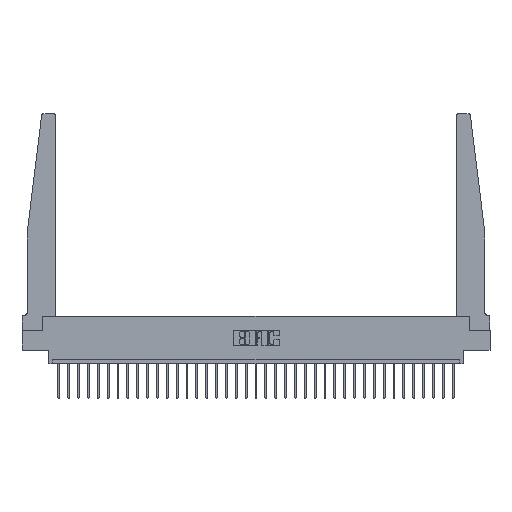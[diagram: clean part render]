
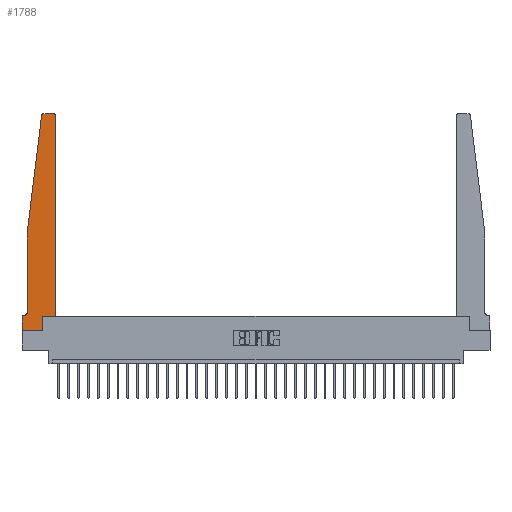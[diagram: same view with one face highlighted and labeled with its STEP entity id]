
A CAD part, top view. The second image highlights one B-rep face of the part: STEP entity #1788.
In plain terms, the highlighted planar face has unit normal (0, 0, 1).
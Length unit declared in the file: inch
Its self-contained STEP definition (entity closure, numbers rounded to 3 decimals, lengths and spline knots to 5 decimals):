
#302 = CARTESIAN_POINT ( 'NONE',  ( 0.065, 0.2375, 0.37 ) ) ;
#506 = DIRECTION ( 'NONE',  ( -0.122, -0.992, 0. ) ) ;
#744 = CARTESIAN_POINT ( 'NONE',  ( 0., 0.1875, 0.37 ) ) ;
#824 = ORIENTED_EDGE ( 'NONE', *, *, #11324, .T. ) ;
#980 = EDGE_LOOP ( 'NONE', ( #824, #16564, #9318, #1576, #23604, #6569, #13724, #20115, #16666, #25024, #13963, #1982 ) ) ;
#1576 = ORIENTED_EDGE ( 'NONE', *, *, #7150, .T. ) ;
#1788 = ADVANCED_FACE ( 'NONE', ( #30078 ), #11517, .T. ) ;
#1829 = EDGE_CURVE ( 'NONE', #10884, #9314, #3560, .T. ) ;
#1982 = ORIENTED_EDGE ( 'NONE', *, *, #28916, .T. ) ;
#1993 = CARTESIAN_POINT ( 'NONE',  ( 0.2605, 0.18, 0.37 ) ) ;
#2552 = VERTEX_POINT ( 'NONE', #6690 ) ;
#2892 = DIRECTION ( 'NONE',  ( -1., 0., 0. ) ) ;
#2907 = VECTOR ( 'NONE', #6822, 39.37008 ) ;
#3037 = VECTOR ( 'NONE', #506, 39.37008 ) ;
#3065 = CARTESIAN_POINT ( 'NONE',  ( 0.395, 2.72, 0.37 ) ) ;
#3560 = LINE ( 'NONE', #10199, #16468 ) ;
#4560 = CARTESIAN_POINT ( 'NONE',  ( 0.24675, 2.72367, 0.37 ) ) ;
#4687 = AXIS2_PLACEMENT_3D ( 'NONE', #11309, #6859, #18734 ) ;
#6132 = VERTEX_POINT ( 'NONE', #302 ) ;
#6374 = CARTESIAN_POINT ( 'NONE',  ( 0.27653, 2.75, 0.37 ) ) ;
#6459 = DIRECTION ( 'NONE',  ( 0., 0., 1. ) ) ;
#6569 = ORIENTED_EDGE ( 'NONE', *, *, #26447, .T. ) ;
#6690 = CARTESIAN_POINT ( 'NONE',  ( 0.395, 2.75, 0.37 ) ) ;
#6822 = DIRECTION ( 'NONE',  ( 1., 0., 0. ) ) ;
#6859 = DIRECTION ( 'NONE',  ( 0., 0., 1. ) ) ;
#6963 = VECTOR ( 'NONE', #16775, 39.37008 ) ;
#7150 = EDGE_CURVE ( 'NONE', #11729, #6132, #19220, .T. ) ;
#7693 = DIRECTION ( 'NONE',  ( 0., 0., -1. ) ) ;
#7741 = CIRCLE ( 'NONE', #8995, 0.03 ) ;
#8168 = LINE ( 'NONE', #14365, #14815 ) ;
#8438 = VERTEX_POINT ( 'NONE', #744 ) ;
#8867 = VECTOR ( 'NONE', #28733, 39.37008 ) ;
#8995 = AXIS2_PLACEMENT_3D ( 'NONE', #3065, #21773, #28898 ) ;
#9023 = CARTESIAN_POINT ( 'NONE',  ( 0.015, 0.1875, 0.37 ) ) ;
#9314 = VERTEX_POINT ( 'NONE', #27834 ) ;
#9318 = ORIENTED_EDGE ( 'NONE', *, *, #17857, .T. ) ;
#10199 = CARTESIAN_POINT ( 'NONE',  ( 0., 0., 0.37 ) ) ;
#10841 = CARTESIAN_POINT ( 'NONE',  ( 0.065, 1.25, 0.37 ) ) ;
#10884 = VERTEX_POINT ( 'NONE', #20030 ) ;
#10976 = CARTESIAN_POINT ( 'NONE',  ( 0.25, 2.75, 0.37 ) ) ;
#11309 = CARTESIAN_POINT ( 'NONE',  ( 0.27653, 2.72, 0.37 ) ) ;
#11324 = EDGE_CURVE ( 'NONE', #2552, #19086, #14134, .T. ) ;
#11517 = PLANE ( 'NONE',  #20085 ) ;
#11729 = VERTEX_POINT ( 'NONE', #29991 ) ;
#11888 = VERTEX_POINT ( 'NONE', #4560 ) ;
#12058 = CARTESIAN_POINT ( 'NONE',  ( 0.065, 1.25, 0.37 ) ) ;
#12326 = VECTOR ( 'NONE', #16571, 39.37008 ) ;
#12417 = CIRCLE ( 'NONE', #30406, 0.05 ) ;
#12482 = LINE ( 'NONE', #25890, #2907 ) ;
#12667 = CARTESIAN_POINT ( 'NONE',  ( 0.065, 0.1875, 0.37 ) ) ;
#13557 = EDGE_CURVE ( 'NONE', #19086, #11888, #15133, .T. ) ;
#13724 = ORIENTED_EDGE ( 'NONE', *, *, #16436, .T. ) ;
#13963 = ORIENTED_EDGE ( 'NONE', *, *, #30093, .T. ) ;
#14134 = LINE ( 'NONE', #10976, #17874 ) ;
#14365 = CARTESIAN_POINT ( 'NONE',  ( 0.2605, 0.18, 0.37 ) ) ;
#14519 = CARTESIAN_POINT ( 'NONE',  ( 0.015, 0.2375, 0.37 ) ) ;
#14535 = DIRECTION ( 'NONE',  ( 1., 0., 0. ) ) ;
#14815 = VECTOR ( 'NONE', #29274, 39.37008 ) ;
#15133 = CIRCLE ( 'NONE', #4687, 0.03 ) ;
#15177 = CARTESIAN_POINT ( 'NONE',  ( 0.425, 2.72, 0.37 ) ) ;
#15567 = CARTESIAN_POINT ( 'NONE',  ( 0.425, 0.18, 0.37 ) ) ;
#15716 = DIRECTION ( 'NONE',  ( -1., 0., 0. ) ) ;
#16058 = VERTEX_POINT ( 'NONE', #15567 ) ;
#16436 = EDGE_CURVE ( 'NONE', #8438, #10884, #18599, .T. ) ;
#16468 = VECTOR ( 'NONE', #14535, 39.37008 ) ;
#16564 = ORIENTED_EDGE ( 'NONE', *, *, #13557, .T. ) ;
#16571 = DIRECTION ( 'NONE',  ( 0., -1., 0. ) ) ;
#16666 = ORIENTED_EDGE ( 'NONE', *, *, #17993, .T. ) ;
#16673 = CARTESIAN_POINT ( 'NONE',  ( 0., 0., 0.37 ) ) ;
#16775 = DIRECTION ( 'NONE',  ( 0., 1., 0. ) ) ;
#17246 = VERTEX_POINT ( 'NONE', #1993 ) ;
#17857 = EDGE_CURVE ( 'NONE', #11888, #11729, #21440, .T. ) ;
#17874 = VECTOR ( 'NONE', #15716, 39.37008 ) ;
#17993 = EDGE_CURVE ( 'NONE', #9314, #17246, #8168, .T. ) ;
#18599 = LINE ( 'NONE', #16673, #12326 ) ;
#18734 = DIRECTION ( 'NONE',  ( 1., 0., 0. ) ) ;
#18933 = DIRECTION ( 'NONE',  ( 1., 0., 0. ) ) ;
#19086 = VERTEX_POINT ( 'NONE', #6374 ) ;
#19220 = LINE ( 'NONE', #12058, #8867 ) ;
#20025 = EDGE_CURVE ( 'NONE', #17246, #16058, #12482, .T. ) ;
#20030 = CARTESIAN_POINT ( 'NONE',  ( 0., 0., 0.37 ) ) ;
#20085 = AXIS2_PLACEMENT_3D ( 'NONE', #20980, #6459, #18933 ) ;
#20115 = ORIENTED_EDGE ( 'NONE', *, *, #1829, .T. ) ;
#20500 = EDGE_CURVE ( 'NONE', #6132, #25500, #12417, .T. ) ;
#20980 = CARTESIAN_POINT ( 'NONE',  ( 0., 0.1875, 0.37 ) ) ;
#21312 = LINE ( 'NONE', #21581, #6963 ) ;
#21440 = LINE ( 'NONE', #10841, #3037 ) ;
#21581 = CARTESIAN_POINT ( 'NONE',  ( 0.425, 0.18, 0.37 ) ) ;
#21773 = DIRECTION ( 'NONE',  ( 0., 0., 1. ) ) ;
#21806 = DIRECTION ( 'NONE',  ( -1., 0., 0. ) ) ;
#23604 = ORIENTED_EDGE ( 'NONE', *, *, #20500, .T. ) ;
#23754 = VECTOR ( 'NONE', #21806, 39.37008 ) ;
#24546 = LINE ( 'NONE', #12667, #23754 ) ;
#25024 = ORIENTED_EDGE ( 'NONE', *, *, #20025, .T. ) ;
#25500 = VERTEX_POINT ( 'NONE', #9023 ) ;
#25890 = CARTESIAN_POINT ( 'NONE',  ( 0.425, 0.18, 0.37 ) ) ;
#26447 = EDGE_CURVE ( 'NONE', #25500, #8438, #24546, .T. ) ;
#27636 = VERTEX_POINT ( 'NONE', #15177 ) ;
#27834 = CARTESIAN_POINT ( 'NONE',  ( 0.2605, 0., 0.37 ) ) ;
#28733 = DIRECTION ( 'NONE',  ( 0., -1., 0. ) ) ;
#28898 = DIRECTION ( 'NONE',  ( 1., 0., 0. ) ) ;
#28916 = EDGE_CURVE ( 'NONE', #27636, #2552, #7741, .T. ) ;
#29274 = DIRECTION ( 'NONE',  ( 0., 1., 0. ) ) ;
#29991 = CARTESIAN_POINT ( 'NONE',  ( 0.065, 1.25, 0.37 ) ) ;
#30078 = FACE_OUTER_BOUND ( 'NONE', #980, .T. ) ;
#30093 = EDGE_CURVE ( 'NONE', #16058, #27636, #21312, .T. ) ;
#30406 = AXIS2_PLACEMENT_3D ( 'NONE', #14519, #7693, #2892 ) ;
